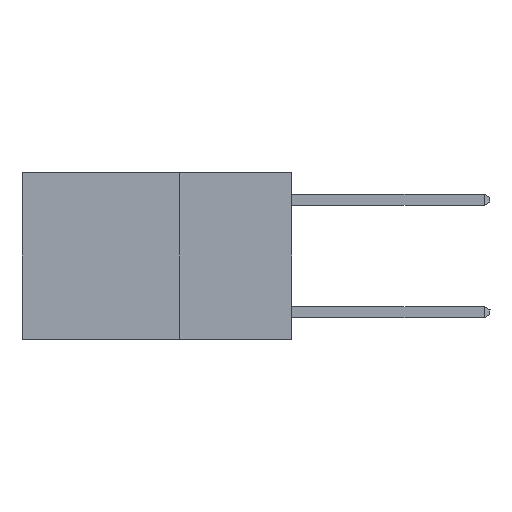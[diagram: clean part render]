
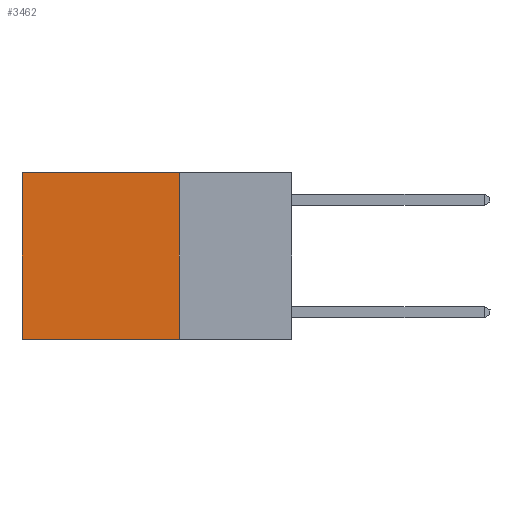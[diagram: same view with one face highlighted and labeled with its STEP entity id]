
A CAD part, left-side view. The second image highlights one B-rep face of the part: STEP entity #3462.
In plain terms, the highlighted planar face has unit normal (-1, 0, 0).
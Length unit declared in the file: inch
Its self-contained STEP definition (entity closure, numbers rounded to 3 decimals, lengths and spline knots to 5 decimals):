
#894 = VERTEX_POINT ( 'NONE', #23778 ) ;
#1186 = EDGE_LOOP ( 'NONE', ( #14069, #14778, #16172, #16378 ) ) ;
#1970 = LINE ( 'NONE', #13235, #24953 ) ;
#2792 = DIRECTION ( 'NONE',  ( 0., 1., 0. ) ) ;
#3380 = DIRECTION ( 'NONE',  ( 1., 0., 0. ) ) ;
#3462 = ADVANCED_FACE ( 'NONE', ( #21951 ), #9622, .F. ) ;
#4642 = EDGE_CURVE ( 'NONE', #15899, #894, #16625, .T. ) ;
#5521 = VECTOR ( 'NONE', #22868, 39.37008 ) ;
#8283 = CARTESIAN_POINT ( 'NONE',  ( 0.2625, 0.25, 0. ) ) ;
#9622 = PLANE ( 'NONE',  #9677 ) ;
#9677 = AXIS2_PLACEMENT_3D ( 'NONE', #26230, #3380, #18052 ) ;
#11544 = CARTESIAN_POINT ( 'NONE',  ( 0.2625, 0.25, 0. ) ) ;
#11939 = CARTESIAN_POINT ( 'NONE',  ( 0.2625, 0.25, 0. ) ) ;
#12487 = VERTEX_POINT ( 'NONE', #21325 ) ;
#13235 = CARTESIAN_POINT ( 'NONE',  ( 0.2625, 0.25, -0.37 ) ) ;
#13344 = EDGE_CURVE ( 'NONE', #16547, #12487, #1970, .T. ) ;
#13400 = VECTOR ( 'NONE', #22792, 39.37008 ) ;
#14069 = ORIENTED_EDGE ( 'NONE', *, *, #25445, .T. ) ;
#14778 = ORIENTED_EDGE ( 'NONE', *, *, #13344, .F. ) ;
#15899 = VERTEX_POINT ( 'NONE', #11939 ) ;
#15944 = LINE ( 'NONE', #8283, #5521 ) ;
#16172 = ORIENTED_EDGE ( 'NONE', *, *, #18008, .F. ) ;
#16378 = ORIENTED_EDGE ( 'NONE', *, *, #4642, .T. ) ;
#16547 = VERTEX_POINT ( 'NONE', #20015 ) ;
#16625 = LINE ( 'NONE', #11544, #21573 ) ;
#17900 = DIRECTION ( 'NONE',  ( 0., 1., 0. ) ) ;
#18008 = EDGE_CURVE ( 'NONE', #15899, #16547, #15944, .T. ) ;
#18052 = DIRECTION ( 'NONE',  ( 0., 0., -1. ) ) ;
#20015 = CARTESIAN_POINT ( 'NONE',  ( 0.2625, 0.25, -0.37 ) ) ;
#21325 = CARTESIAN_POINT ( 'NONE',  ( 0.2625, 0.6, -0.37 ) ) ;
#21573 = VECTOR ( 'NONE', #17900, 39.37008 ) ;
#21951 = FACE_OUTER_BOUND ( 'NONE', #1186, .T. ) ;
#22792 = DIRECTION ( 'NONE',  ( 0., 0., -1. ) ) ;
#22868 = DIRECTION ( 'NONE',  ( 0., 0., -1. ) ) ;
#23778 = CARTESIAN_POINT ( 'NONE',  ( 0.2625, 0.6, 0. ) ) ;
#24547 = LINE ( 'NONE', #26788, #13400 ) ;
#24953 = VECTOR ( 'NONE', #2792, 39.37008 ) ;
#25445 = EDGE_CURVE ( 'NONE', #894, #12487, #24547, .T. ) ;
#26230 = CARTESIAN_POINT ( 'NONE',  ( 0.2625, 0.25, 0. ) ) ;
#26788 = CARTESIAN_POINT ( 'NONE',  ( 0.2625, 0.6, 0. ) ) ;
